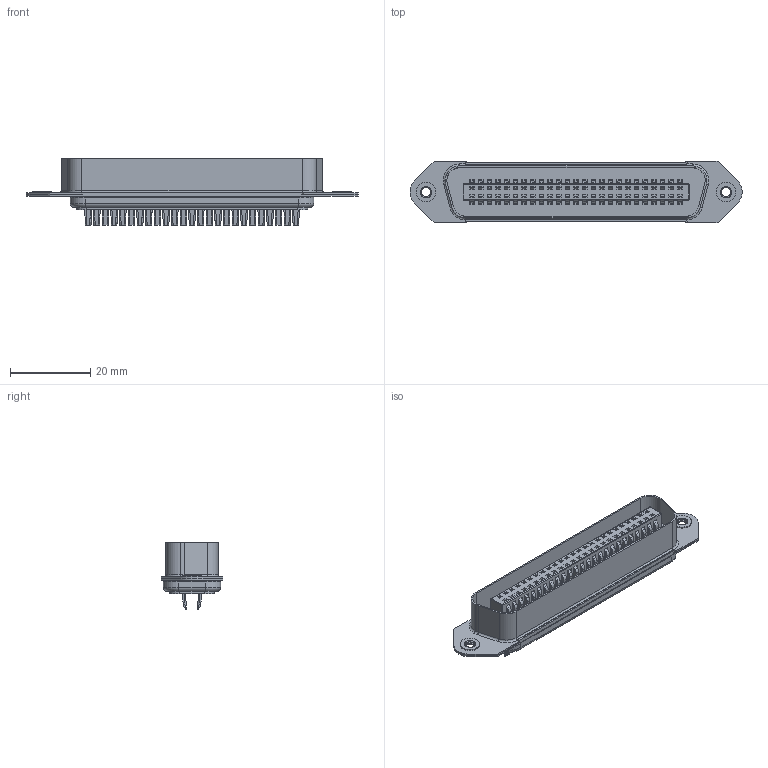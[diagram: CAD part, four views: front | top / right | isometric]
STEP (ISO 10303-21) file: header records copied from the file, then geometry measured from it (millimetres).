
FILE_DESCRIPTION (( 'STEP AP203' ), '1' );
FILE_NAME ('B57-150-622-302.STEP', '2020-06-24T12:40:54', ( '' ), ( '' ), 'SwSTEP 2.0', 'SolidWorks 2020', '' );
FILE_SCHEMA (( 'CONFIG_CONTROL_DESIGN' ));
Length unit declared in the file: millimetre
Products named in the file (6): B57 Back Shell_50 Position; B57 Front Shell MALE_50 Position UP; B57 Contacts MALE_50 Position SOLDER; B57-150-622-302; B57 Housing Insert MALE_50 Position UP; B57 Rivet_STR THREAD
Assembly tree (6 placements, depth 2):
  B57-150-622-302
    B57 Back Shell_50 Position
    B57 Rivet_STR THREAD  x2
    B57 Housing Insert MALE_50 Position UP
    B57 Front Shell MALE_50 Position UP
    B57 Contacts MALE_50 Position SOLDER
Bounding box: 82.83 x 15.3 x 16.57 mm (x, y, z)
Volume: 5890.2 mm3; surface area: 14624.1 mm2
Topology: 55 solids, 55 shells, 5243 faces, 14921 edges, 9488 vertices
Faces by surface type: plane 3771, cylinder 1230, sphere 204, torus 32, bspline 6
Entity records: 168650 total; most frequent: CARTESIAN_POINT 33193, ORIENTED_EDGE 29350, DIRECTION 26562, EDGE_CURVE 14675, LINE 11758, VECTOR 11758, VERTEX_POINT 9460, AXIS2_PLACEMENT_3D 7402
